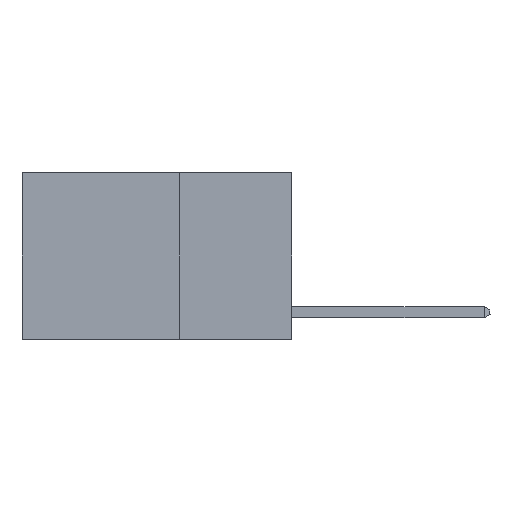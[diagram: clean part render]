
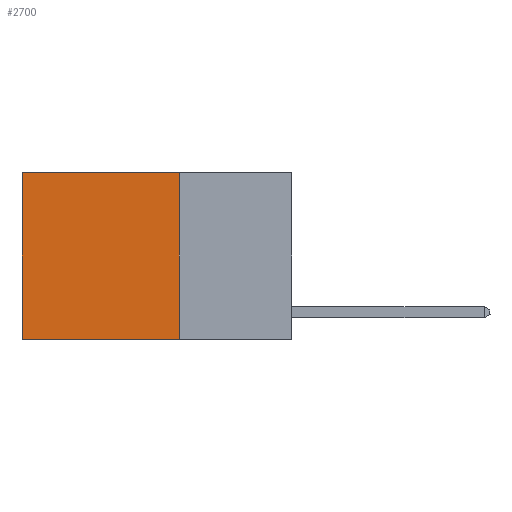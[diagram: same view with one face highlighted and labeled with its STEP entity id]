
A CAD part, left-side view. The second image highlights one B-rep face of the part: STEP entity #2700.
In plain terms, the highlighted planar face has unit normal (-1, 0, 0).
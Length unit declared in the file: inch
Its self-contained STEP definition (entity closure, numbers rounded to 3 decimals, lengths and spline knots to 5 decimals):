
#192 = CARTESIAN_POINT ( 'NONE',  ( 0.2625, 0.25, 0. ) ) ;
#255 = EDGE_LOOP ( 'NONE', ( #8213, #6265, #4678, #2390 ) ) ;
#320 = FACE_OUTER_BOUND ( 'NONE', #255, .T. ) ;
#784 = CARTESIAN_POINT ( 'NONE',  ( 0.2625, 0.25, -0.37 ) ) ;
#1079 = LINE ( 'NONE', #5375, #8529 ) ;
#1262 = VERTEX_POINT ( 'NONE', #6066 ) ;
#1446 = EDGE_CURVE ( 'NONE', #1262, #9140, #2789, .T. ) ;
#1749 = CARTESIAN_POINT ( 'NONE',  ( 0.2625, 0.25, -0.37 ) ) ;
#1982 = EDGE_CURVE ( 'NONE', #9631, #3641, #7759, .T. ) ;
#2390 = ORIENTED_EDGE ( 'NONE', *, *, #7395, .T. ) ;
#2700 = ADVANCED_FACE ( 'NONE', ( #320 ), #10386, .F. ) ;
#2789 = LINE ( 'NONE', #192, #10704 ) ;
#2984 = DIRECTION ( 'NONE',  ( 0., 0., -1. ) ) ;
#3641 = VERTEX_POINT ( 'NONE', #11712 ) ;
#3880 = CARTESIAN_POINT ( 'NONE',  ( 0.2625, 0.25, 0. ) ) ;
#4051 = VECTOR ( 'NONE', #5430, 39.37008 ) ;
#4678 = ORIENTED_EDGE ( 'NONE', *, *, #1446, .F. ) ;
#4905 = AXIS2_PLACEMENT_3D ( 'NONE', #3880, #6511, #2984 ) ;
#5375 = CARTESIAN_POINT ( 'NONE',  ( 0.2625, 0.25, 0. ) ) ;
#5430 = DIRECTION ( 'NONE',  ( 0., 1., 0. ) ) ;
#5843 = CARTESIAN_POINT ( 'NONE',  ( 0.2625, 0.6, 0. ) ) ;
#6066 = CARTESIAN_POINT ( 'NONE',  ( 0.2625, 0.25, 0. ) ) ;
#6265 = ORIENTED_EDGE ( 'NONE', *, *, #10443, .F. ) ;
#6511 = DIRECTION ( 'NONE',  ( 1., 0., 0. ) ) ;
#6576 = DIRECTION ( 'NONE',  ( 0., 0., -1. ) ) ;
#6847 = DIRECTION ( 'NONE',  ( 0., 0., -1. ) ) ;
#7395 = EDGE_CURVE ( 'NONE', #1262, #9631, #1079, .T. ) ;
#7759 = LINE ( 'NONE', #9331, #8835 ) ;
#8034 = DIRECTION ( 'NONE',  ( 0., 1., 0. ) ) ;
#8213 = ORIENTED_EDGE ( 'NONE', *, *, #1982, .T. ) ;
#8529 = VECTOR ( 'NONE', #8034, 39.37008 ) ;
#8835 = VECTOR ( 'NONE', #6847, 39.37008 ) ;
#9140 = VERTEX_POINT ( 'NONE', #784 ) ;
#9331 = CARTESIAN_POINT ( 'NONE',  ( 0.2625, 0.6, 0. ) ) ;
#9631 = VERTEX_POINT ( 'NONE', #5843 ) ;
#10007 = LINE ( 'NONE', #1749, #4051 ) ;
#10386 = PLANE ( 'NONE',  #4905 ) ;
#10443 = EDGE_CURVE ( 'NONE', #9140, #3641, #10007, .T. ) ;
#10704 = VECTOR ( 'NONE', #6576, 39.37008 ) ;
#11712 = CARTESIAN_POINT ( 'NONE',  ( 0.2625, 0.6, -0.37 ) ) ;
